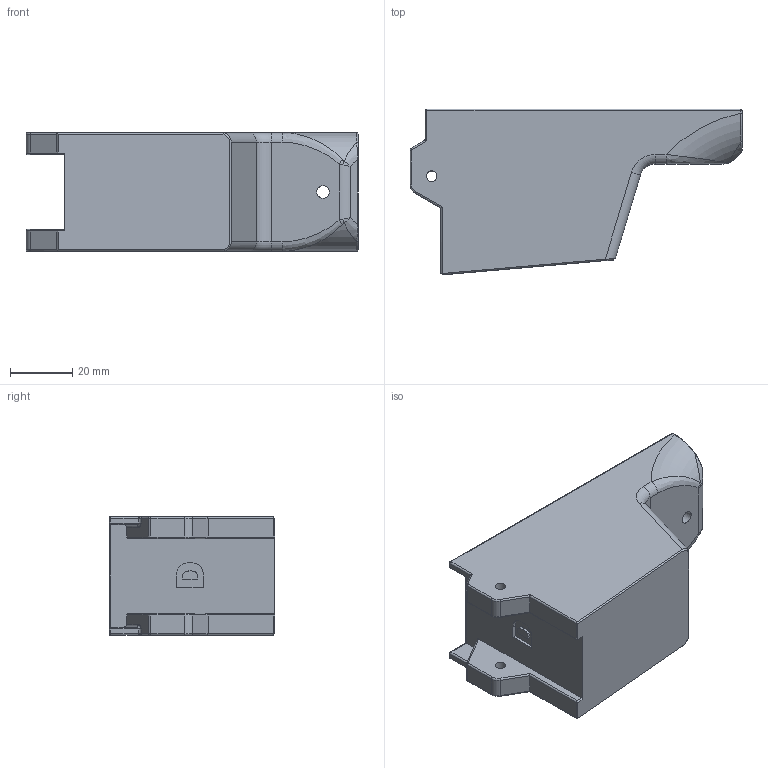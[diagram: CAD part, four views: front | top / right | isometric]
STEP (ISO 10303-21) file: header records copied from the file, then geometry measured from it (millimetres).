
FILE_DESCRIPTION(/* description */ (''),/* implementation_level */ '2;1');
FILE_NAME(/* author */ (''),/* organization */ (''),/* preprocessor_version */ 'ST-DEVELOPER v15.2',/* originating_system */ 'Autodesk Translator Framework v2.0.0.5431',/* authorisation */ '');
FILE_SCHEMA (('AUTOMOTIVE_DESIGN { 1 0 10303 214 3 1 1 }'));
Length unit declared in the file: centimetre
Products named in the file (1): MOD9 QUICK PRINT MAGWELL
Bounding box: 106.51 x 53.17 x 38 mm (x, y, z)
Volume: 135607.1 mm3; surface area: 19554.7 mm2
Topology: 1 solids, 1 shells, 154 faces, 379 edges, 225 vertices
Faces by surface type: cylinder 50, bspline 45, plane 44, torus 9, sphere 6
Full cylindrical faces by diameter (mm): 3.4 x2, 4 x2
Entity records: 5425 total; most frequent: CARTESIAN_POINT 2039, ORIENTED_EDGE 740, DIRECTION 620, EDGE_CURVE 370, VERTEX_POINT 225, AXIS2_PLACEMENT_3D 221, LINE 178, VECTOR 178
